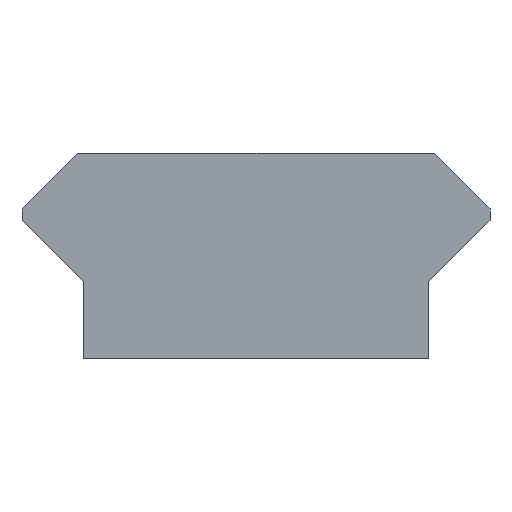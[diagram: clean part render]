
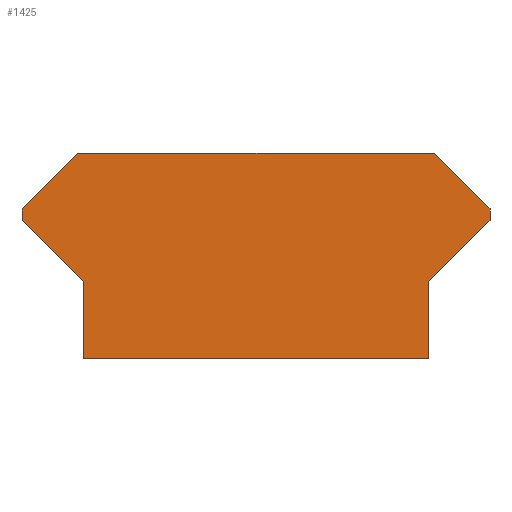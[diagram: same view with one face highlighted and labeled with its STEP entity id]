
A CAD part, front view. The second image highlights one B-rep face of the part: STEP entity #1425.
In plain terms, the highlighted planar face has unit normal (0, -1, 0).
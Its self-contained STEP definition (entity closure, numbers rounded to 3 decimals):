
#19=FACE_OUTER_BOUND('',#91,.T.);
#91=EDGE_LOOP('',(#985,#986,#987,#988,#989,#990,#991,#992,#993,#994));
#159=LINE('',#1939,#369);
#203=LINE('',#2027,#413);
#206=LINE('',#2033,#416);
#209=LINE('',#2039,#419);
#212=LINE('',#2045,#422);
#213=LINE('',#2047,#423);
#214=LINE('',#2049,#424);
#215=LINE('',#2051,#425);
#216=LINE('',#2053,#426);
#217=LINE('',#2054,#427);
#369=VECTOR('',#1583,10.);
#413=VECTOR('',#1629,10.);
#416=VECTOR('',#1634,10.);
#419=VECTOR('',#1639,10.);
#422=VECTOR('',#1644,10.);
#423=VECTOR('',#1645,10.);
#424=VECTOR('',#1646,10.);
#425=VECTOR('',#1647,10.);
#426=VECTOR('',#1648,10.);
#427=VECTOR('',#1649,10.);
#579=VERTEX_POINT('',#1937);
#580=VERTEX_POINT('',#1938);
#623=VERTEX_POINT('',#2026);
#625=VERTEX_POINT('',#2032);
#627=VERTEX_POINT('',#2038);
#629=VERTEX_POINT('',#2044);
#630=VERTEX_POINT('',#2046);
#631=VERTEX_POINT('',#2048);
#632=VERTEX_POINT('',#2050);
#633=VERTEX_POINT('',#2052);
#719=EDGE_CURVE('',#579,#580,#159,.T.);
#763=EDGE_CURVE('',#623,#579,#203,.T.);
#766=EDGE_CURVE('',#625,#623,#206,.T.);
#769=EDGE_CURVE('',#627,#625,#209,.T.);
#772=EDGE_CURVE('',#629,#580,#212,.T.);
#773=EDGE_CURVE('',#630,#629,#213,.T.);
#774=EDGE_CURVE('',#631,#630,#214,.T.);
#775=EDGE_CURVE('',#631,#632,#215,.T.);
#776=EDGE_CURVE('',#632,#633,#216,.T.);
#777=EDGE_CURVE('',#633,#627,#217,.T.);
#985=ORIENTED_EDGE('',*,*,#719,.T.);
#986=ORIENTED_EDGE('',*,*,#772,.F.);
#987=ORIENTED_EDGE('',*,*,#773,.F.);
#988=ORIENTED_EDGE('',*,*,#774,.F.);
#989=ORIENTED_EDGE('',*,*,#775,.T.);
#990=ORIENTED_EDGE('',*,*,#776,.T.);
#991=ORIENTED_EDGE('',*,*,#777,.T.);
#992=ORIENTED_EDGE('',*,*,#769,.T.);
#993=ORIENTED_EDGE('',*,*,#766,.T.);
#994=ORIENTED_EDGE('',*,*,#763,.T.);
#1353=PLANE('',#1511);
#1425=ADVANCED_FACE('',(#19),#1353,.F.);
#1511=AXIS2_PLACEMENT_3D('',#2043,#1642,#1643);
#1583=DIRECTION('',(0.,0.,1.));
#1629=DIRECTION('',(0.707,0.,0.707));
#1634=DIRECTION('',(0.,0.,1.));
#1639=DIRECTION('',(1.,0.,0.));
#1642=DIRECTION('center_axis',(0.,1.,0.));
#1643=DIRECTION('ref_axis',(0.,0.,1.));
#1644=DIRECTION('',(0.707,0.,-0.707));
#1645=DIRECTION('',(1.,0.,0.));
#1646=DIRECTION('',(0.707,0.,0.707));
#1647=DIRECTION('',(0.,0.,-1.));
#1648=DIRECTION('',(0.707,0.,-0.707));
#1649=DIRECTION('',(0.,0.,-1.));
#1937=CARTESIAN_POINT('',(10.605,-12.347,-16.142));
#1938=CARTESIAN_POINT('',(10.605,-12.347,-15.608));
#1939=CARTESIAN_POINT('',(10.605,-12.347,-16.675));
#2026=CARTESIAN_POINT('',(7.836,-12.347,-18.91));
#2027=CARTESIAN_POINT('',(7.553,-12.347,-19.193));
#2032=CARTESIAN_POINT('',(7.836,-12.347,-22.403));
#2033=CARTESIAN_POINT('',(7.836,-12.347,-18.205));
#2038=CARTESIAN_POINT('',(-7.836,-12.347,-22.403));
#2039=CARTESIAN_POINT('',(-3.918,-12.347,-22.403));
#2043=CARTESIAN_POINT('Origin',(-10.605,-12.347,-16.078));
#2044=CARTESIAN_POINT('',(8.077,-12.347,-13.081));
#2045=CARTESIAN_POINT('',(4.867,-12.347,-9.871));
#2046=CARTESIAN_POINT('',(-8.077,-12.347,-13.081));
#2047=CARTESIAN_POINT('',(-9.341,-12.347,-13.081));
#2048=CARTESIAN_POINT('',(-10.605,-12.347,-15.608));
#2049=CARTESIAN_POINT('',(-10.17,-12.347,-15.173));
#2050=CARTESIAN_POINT('',(-10.605,-12.347,-16.142));
#2051=CARTESIAN_POINT('',(-10.605,-12.347,-16.675));
#2052=CARTESIAN_POINT('',(-7.836,-12.347,-18.91));
#2053=CARTESIAN_POINT('',(-7.001,-12.347,-19.745));
#2054=CARTESIAN_POINT('',(-7.836,-12.347,-18.205));
